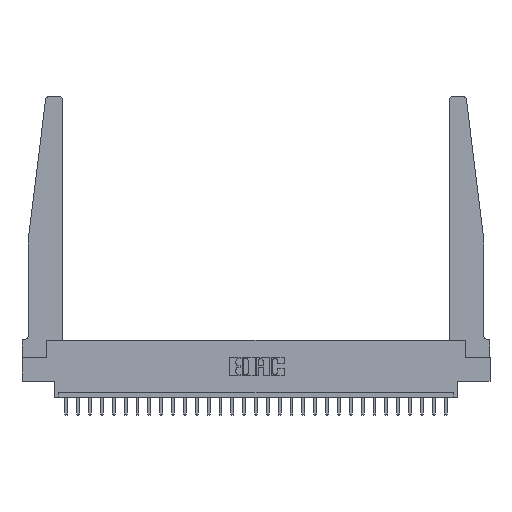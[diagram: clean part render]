
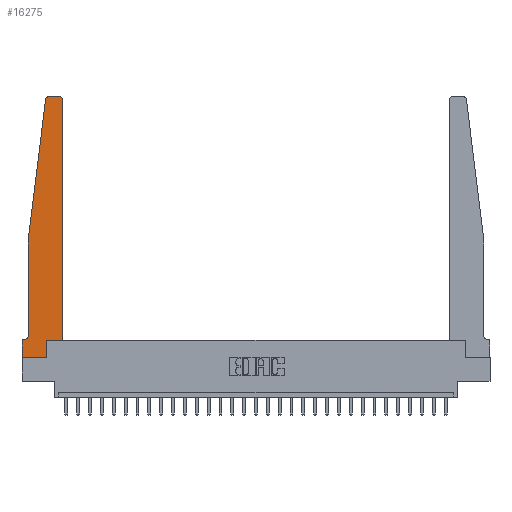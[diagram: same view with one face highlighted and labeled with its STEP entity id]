
A CAD part, top view. The second image highlights one B-rep face of the part: STEP entity #16275.
In plain terms, the highlighted planar face has unit normal (0, 0, 1).
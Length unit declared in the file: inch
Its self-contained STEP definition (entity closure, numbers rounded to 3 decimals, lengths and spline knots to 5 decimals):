
#107 = VECTOR ( 'NONE', #19030, 39.37008 ) ;
#192 = ORIENTED_EDGE ( 'NONE', *, *, #8571, .T. ) ;
#457 = CARTESIAN_POINT ( 'NONE',  ( 0.015, 0.1875, 0.37 ) ) ;
#466 = AXIS2_PLACEMENT_3D ( 'NONE', #8363, #1892, #5766 ) ;
#715 = CARTESIAN_POINT ( 'NONE',  ( 0.24675, 2.72367, 0.37 ) ) ;
#1109 = CARTESIAN_POINT ( 'NONE',  ( 0., 0., 0.37 ) ) ;
#1258 = VERTEX_POINT ( 'NONE', #2910 ) ;
#1892 = DIRECTION ( 'NONE',  ( 0., 0., 1. ) ) ;
#2033 = ORIENTED_EDGE ( 'NONE', *, *, #12424, .T. ) ;
#2462 = CARTESIAN_POINT ( 'NONE',  ( 0.425, 0.18, 0.37 ) ) ;
#2910 = CARTESIAN_POINT ( 'NONE',  ( 0.2605, 0., 0.37 ) ) ;
#2973 = CARTESIAN_POINT ( 'NONE',  ( 0.065, 1.25, 0.37 ) ) ;
#3128 = ORIENTED_EDGE ( 'NONE', *, *, #16028, .T. ) ;
#3202 = ORIENTED_EDGE ( 'NONE', *, *, #11567, .T. ) ;
#3296 = VECTOR ( 'NONE', #17550, 39.37008 ) ;
#3396 = DIRECTION ( 'NONE',  ( 0., 0., 1. ) ) ;
#3544 = DIRECTION ( 'NONE',  ( 0., 0., -1. ) ) ;
#3626 = ORIENTED_EDGE ( 'NONE', *, *, #14707, .T. ) ;
#4863 = DIRECTION ( 'NONE',  ( 1., 0., 0. ) ) ;
#4907 = CARTESIAN_POINT ( 'NONE',  ( 0.065, 0.2375, 0.37 ) ) ;
#4913 = DIRECTION ( 'NONE',  ( 1., 0., 0. ) ) ;
#5368 = CARTESIAN_POINT ( 'NONE',  ( 0.2605, 0.18, 0.37 ) ) ;
#5499 = EDGE_CURVE ( 'NONE', #1258, #18399, #24180, .T. ) ;
#5766 = DIRECTION ( 'NONE',  ( 1., 0., 0. ) ) ;
#6048 = EDGE_CURVE ( 'NONE', #26764, #15921, #20827, .T. ) ;
#6206 = VECTOR ( 'NONE', #4913, 39.37008 ) ;
#6621 = LINE ( 'NONE', #9218, #26356 ) ;
#6847 = LINE ( 'NONE', #17003, #6206 ) ;
#6938 = CARTESIAN_POINT ( 'NONE',  ( 0.425, 0.18, 0.37 ) ) ;
#6942 = VECTOR ( 'NONE', #7706, 39.37008 ) ;
#7113 = VERTEX_POINT ( 'NONE', #22443 ) ;
#7706 = DIRECTION ( 'NONE',  ( 0., -1., 0. ) ) ;
#7991 = DIRECTION ( 'NONE',  ( 1., 0., 0. ) ) ;
#8363 = CARTESIAN_POINT ( 'NONE',  ( 0., 0.1875, 0.37 ) ) ;
#8406 = ORIENTED_EDGE ( 'NONE', *, *, #6048, .T. ) ;
#8571 = EDGE_CURVE ( 'NONE', #18892, #26764, #14804, .T. ) ;
#8579 = LINE ( 'NONE', #10343, #107 ) ;
#8754 = VECTOR ( 'NONE', #22119, 39.37008 ) ;
#8819 = VERTEX_POINT ( 'NONE', #17590 ) ;
#9074 = DIRECTION ( 'NONE',  ( -1., 0., 0. ) ) ;
#9218 = CARTESIAN_POINT ( 'NONE',  ( 0.25, 2.75, 0.37 ) ) ;
#9345 = ORIENTED_EDGE ( 'NONE', *, *, #21221, .T. ) ;
#9683 = EDGE_CURVE ( 'NONE', #18399, #22699, #25609, .T. ) ;
#9709 = CARTESIAN_POINT ( 'NONE',  ( 0.395, 2.72, 0.37 ) ) ;
#10044 = CIRCLE ( 'NONE', #10955, 0.05 ) ;
#10093 = CARTESIAN_POINT ( 'NONE',  ( 0.2605, 0.18, 0.37 ) ) ;
#10343 = CARTESIAN_POINT ( 'NONE',  ( 0.425, 0.18, 0.37 ) ) ;
#10955 = AXIS2_PLACEMENT_3D ( 'NONE', #20430, #3544, #14242 ) ;
#11024 = FACE_OUTER_BOUND ( 'NONE', #16174, .T. ) ;
#11303 = VERTEX_POINT ( 'NONE', #4907 ) ;
#11567 = EDGE_CURVE ( 'NONE', #22699, #16390, #8579, .T. ) ;
#12424 = EDGE_CURVE ( 'NONE', #8819, #1258, #6847, .T. ) ;
#12828 = ORIENTED_EDGE ( 'NONE', *, *, #9683, .T. ) ;
#13478 = VECTOR ( 'NONE', #4863, 39.37008 ) ;
#13505 = VECTOR ( 'NONE', #24951, 39.37008 ) ;
#14189 = CARTESIAN_POINT ( 'NONE',  ( 0.27653, 2.75, 0.37 ) ) ;
#14242 = DIRECTION ( 'NONE',  ( -1., 0., 0. ) ) ;
#14428 = DIRECTION ( 'NONE',  ( 0., 0., 1. ) ) ;
#14707 = EDGE_CURVE ( 'NONE', #7113, #8819, #15817, .T. ) ;
#14804 = CIRCLE ( 'NONE', #23148, 0.03 ) ;
#15117 = EDGE_CURVE ( 'NONE', #11303, #25617, #10044, .T. ) ;
#15211 = ORIENTED_EDGE ( 'NONE', *, *, #22025, .T. ) ;
#15817 = LINE ( 'NONE', #1109, #6942 ) ;
#15921 = VERTEX_POINT ( 'NONE', #21879 ) ;
#16028 = EDGE_CURVE ( 'NONE', #19321, #18892, #6621, .T. ) ;
#16174 = EDGE_LOOP ( 'NONE', ( #3128, #192, #8406, #15211, #17142, #17734, #3626, #2033, #16749, #12828, #3202, #9345 ) ) ;
#16275 = ADVANCED_FACE ( 'NONE', ( #11024 ), #20719, .T. ) ;
#16298 = LINE ( 'NONE', #22492, #16506 ) ;
#16390 = VERTEX_POINT ( 'NONE', #21003 ) ;
#16506 = VECTOR ( 'NONE', #20414, 39.37008 ) ;
#16711 = CARTESIAN_POINT ( 'NONE',  ( 0.065, 1.25, 0.37 ) ) ;
#16749 = ORIENTED_EDGE ( 'NONE', *, *, #5499, .T. ) ;
#17003 = CARTESIAN_POINT ( 'NONE',  ( 0., 0., 0.37 ) ) ;
#17142 = ORIENTED_EDGE ( 'NONE', *, *, #15117, .T. ) ;
#17550 = DIRECTION ( 'NONE',  ( 0., -1., 0. ) ) ;
#17590 = CARTESIAN_POINT ( 'NONE',  ( 0., 0., 0.37 ) ) ;
#17734 = ORIENTED_EDGE ( 'NONE', *, *, #21285, .T. ) ;
#18399 = VERTEX_POINT ( 'NONE', #10093 ) ;
#18892 = VERTEX_POINT ( 'NONE', #14189 ) ;
#19030 = DIRECTION ( 'NONE',  ( 0., 1., 0. ) ) ;
#19321 = VERTEX_POINT ( 'NONE', #20476 ) ;
#19605 = CIRCLE ( 'NONE', #21799, 0.03 ) ;
#20414 = DIRECTION ( 'NONE',  ( -1., 0., 0. ) ) ;
#20430 = CARTESIAN_POINT ( 'NONE',  ( 0.015, 0.2375, 0.37 ) ) ;
#20476 = CARTESIAN_POINT ( 'NONE',  ( 0.395, 2.75, 0.37 ) ) ;
#20719 = PLANE ( 'NONE',  #466 ) ;
#20827 = LINE ( 'NONE', #16711, #13505 ) ;
#21003 = CARTESIAN_POINT ( 'NONE',  ( 0.425, 2.72, 0.37 ) ) ;
#21221 = EDGE_CURVE ( 'NONE', #16390, #19321, #19605, .T. ) ;
#21285 = EDGE_CURVE ( 'NONE', #25617, #7113, #16298, .T. ) ;
#21799 = AXIS2_PLACEMENT_3D ( 'NONE', #9709, #3396, #21962 ) ;
#21879 = CARTESIAN_POINT ( 'NONE',  ( 0.065, 1.25, 0.37 ) ) ;
#21962 = DIRECTION ( 'NONE',  ( 1., 0., 0. ) ) ;
#22025 = EDGE_CURVE ( 'NONE', #15921, #11303, #23310, .T. ) ;
#22119 = DIRECTION ( 'NONE',  ( 0., 1., 0. ) ) ;
#22443 = CARTESIAN_POINT ( 'NONE',  ( 0., 0.1875, 0.37 ) ) ;
#22492 = CARTESIAN_POINT ( 'NONE',  ( 0.065, 0.1875, 0.37 ) ) ;
#22699 = VERTEX_POINT ( 'NONE', #2462 ) ;
#23148 = AXIS2_PLACEMENT_3D ( 'NONE', #26416, #14428, #7991 ) ;
#23310 = LINE ( 'NONE', #2973, #3296 ) ;
#24180 = LINE ( 'NONE', #5368, #8754 ) ;
#24951 = DIRECTION ( 'NONE',  ( -0.122, -0.992, 0. ) ) ;
#25609 = LINE ( 'NONE', #6938, #13478 ) ;
#25617 = VERTEX_POINT ( 'NONE', #457 ) ;
#26356 = VECTOR ( 'NONE', #9074, 39.37008 ) ;
#26416 = CARTESIAN_POINT ( 'NONE',  ( 0.27653, 2.72, 0.37 ) ) ;
#26764 = VERTEX_POINT ( 'NONE', #715 ) ;
